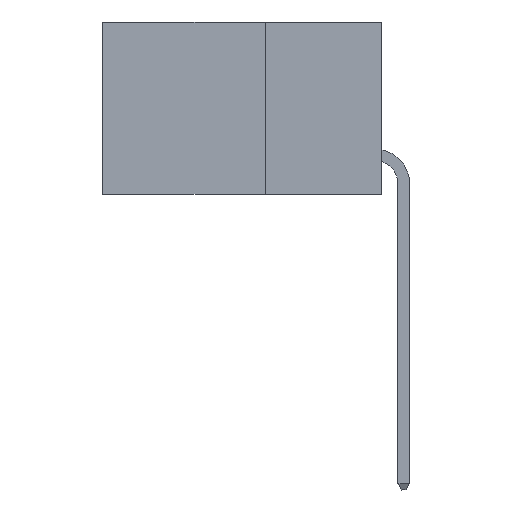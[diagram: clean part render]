
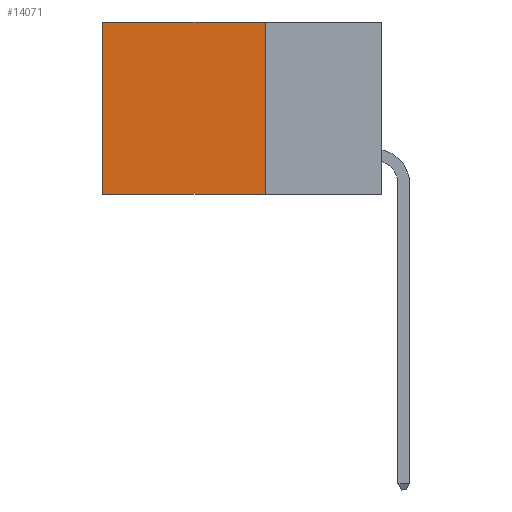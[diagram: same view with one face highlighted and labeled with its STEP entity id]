
A CAD part, left-side view. The second image highlights one B-rep face of the part: STEP entity #14071.
In plain terms, the highlighted planar face has unit normal (-1, 0, 0).
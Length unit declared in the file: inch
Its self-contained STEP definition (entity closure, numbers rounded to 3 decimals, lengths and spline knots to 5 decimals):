
#2569 = LINE ( 'NONE', #5654, #15372 ) ;
#2806 = EDGE_CURVE ( 'NONE', #9283, #13576, #13533, .T. ) ;
#3237 = FACE_OUTER_BOUND ( 'NONE', #12071, .T. ) ;
#4742 = CARTESIAN_POINT ( 'NONE',  ( 0.2875, 0.25, 0. ) ) ;
#4757 = VECTOR ( 'NONE', #6378, 39.37008 ) ;
#5025 = CARTESIAN_POINT ( 'NONE',  ( 0.2875, 0.25, 0. ) ) ;
#5654 = CARTESIAN_POINT ( 'NONE',  ( 0.2875, 0.25, -0.37 ) ) ;
#6378 = DIRECTION ( 'NONE',  ( 0., 0., -1. ) ) ;
#8054 = ORIENTED_EDGE ( 'NONE', *, *, #11824, .T. ) ;
#8508 = CARTESIAN_POINT ( 'NONE',  ( 0.2875, 0.25, -0.37 ) ) ;
#9283 = VERTEX_POINT ( 'NONE', #11019 ) ;
#9663 = ORIENTED_EDGE ( 'NONE', *, *, #2806, .T. ) ;
#9751 = DIRECTION ( 'NONE',  ( 0., 0., -1. ) ) ;
#9890 = LINE ( 'NONE', #4742, #4757 ) ;
#10747 = VERTEX_POINT ( 'NONE', #19318 ) ;
#11019 = CARTESIAN_POINT ( 'NONE',  ( 0.2875, 0.25, 0. ) ) ;
#11230 = PLANE ( 'NONE',  #17773 ) ;
#11285 = DIRECTION ( 'NONE',  ( 0., 0., -1. ) ) ;
#11400 = EDGE_CURVE ( 'NONE', #11971, #10747, #2569, .T. ) ;
#11824 = EDGE_CURVE ( 'NONE', #13576, #10747, #11832, .T. ) ;
#11832 = LINE ( 'NONE', #18747, #18837 ) ;
#11971 = VERTEX_POINT ( 'NONE', #8508 ) ;
#12071 = EDGE_LOOP ( 'NONE', ( #8054, #12575, #16527, #9663 ) ) ;
#12397 = EDGE_CURVE ( 'NONE', #9283, #11971, #9890, .T. ) ;
#12575 = ORIENTED_EDGE ( 'NONE', *, *, #11400, .F. ) ;
#13533 = LINE ( 'NONE', #17947, #17486 ) ;
#13576 = VERTEX_POINT ( 'NONE', #18832 ) ;
#14071 = ADVANCED_FACE ( 'NONE', ( #3237 ), #11230, .F. ) ;
#15372 = VECTOR ( 'NONE', #17824, 39.37008 ) ;
#16527 = ORIENTED_EDGE ( 'NONE', *, *, #12397, .F. ) ;
#17486 = VECTOR ( 'NONE', #19496, 39.37008 ) ;
#17773 = AXIS2_PLACEMENT_3D ( 'NONE', #5025, #18755, #9751 ) ;
#17824 = DIRECTION ( 'NONE',  ( 0., 1., 0. ) ) ;
#17947 = CARTESIAN_POINT ( 'NONE',  ( 0.2875, 0.25, 0. ) ) ;
#18747 = CARTESIAN_POINT ( 'NONE',  ( 0.2875, 0.6, 0. ) ) ;
#18755 = DIRECTION ( 'NONE',  ( 1., 0., 0. ) ) ;
#18832 = CARTESIAN_POINT ( 'NONE',  ( 0.2875, 0.6, 0. ) ) ;
#18837 = VECTOR ( 'NONE', #11285, 39.37008 ) ;
#19318 = CARTESIAN_POINT ( 'NONE',  ( 0.2875, 0.6, -0.37 ) ) ;
#19496 = DIRECTION ( 'NONE',  ( 0., 1., 0. ) ) ;
